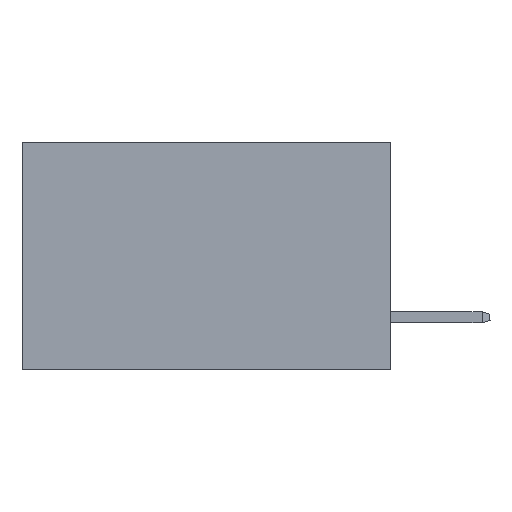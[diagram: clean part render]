
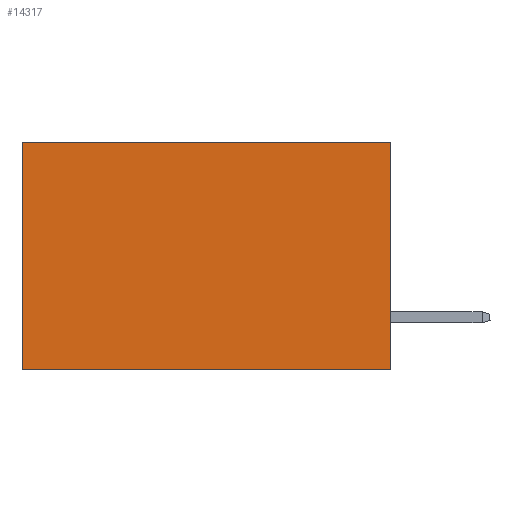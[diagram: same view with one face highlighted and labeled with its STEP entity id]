
A CAD part, left-side view. The second image highlights one B-rep face of the part: STEP entity #14317.
In plain terms, the highlighted planar face has unit normal (-1, 0, 0).
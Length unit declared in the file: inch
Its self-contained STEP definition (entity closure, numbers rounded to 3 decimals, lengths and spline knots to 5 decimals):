
#1165 = EDGE_CURVE ( 'NONE', #21384, #20800, #18190, .T. ) ;
#1478 = CARTESIAN_POINT ( 'NONE',  ( 0.2875, 0., 0. ) ) ;
#1890 = FACE_OUTER_BOUND ( 'NONE', #25519, .T. ) ;
#4915 = ORIENTED_EDGE ( 'NONE', *, *, #15738, .F. ) ;
#5184 = DIRECTION ( 'NONE',  ( 1., 0., 0. ) ) ;
#6334 = CARTESIAN_POINT ( 'NONE',  ( 0.2875, 0.6, 0. ) ) ;
#7703 = LINE ( 'NONE', #1478, #8691 ) ;
#8682 = VERTEX_POINT ( 'NONE', #22305 ) ;
#8691 = VECTOR ( 'NONE', #23626, 39.37008 ) ;
#9020 = ORIENTED_EDGE ( 'NONE', *, *, #1165, .T. ) ;
#9028 = PLANE ( 'NONE',  #11332 ) ;
#10023 = CARTESIAN_POINT ( 'NONE',  ( 0.2875, 0., 0. ) ) ;
#10754 = CARTESIAN_POINT ( 'NONE',  ( 0.2875, 0., 0. ) ) ;
#11332 = AXIS2_PLACEMENT_3D ( 'NONE', #13520, #5184, #19682 ) ;
#11790 = ORIENTED_EDGE ( 'NONE', *, *, #26344, .F. ) ;
#11965 = CARTESIAN_POINT ( 'NONE',  ( 0.2875, 0.6, 0. ) ) ;
#12407 = VECTOR ( 'NONE', #26086, 39.37008 ) ;
#13243 = ORIENTED_EDGE ( 'NONE', *, *, #21626, .T. ) ;
#13520 = CARTESIAN_POINT ( 'NONE',  ( 0.2875, 0., 0. ) ) ;
#14317 = ADVANCED_FACE ( 'NONE', ( #1890 ), #9028, .F. ) ;
#14984 = LINE ( 'NONE', #23029, #24853 ) ;
#15738 = EDGE_CURVE ( 'NONE', #8682, #24709, #14984, .T. ) ;
#15828 = LINE ( 'NONE', #11965, #16168 ) ;
#16168 = VECTOR ( 'NONE', #22227, 39.37008 ) ;
#16322 = CARTESIAN_POINT ( 'NONE',  ( 0.2875, 0.6, -0.37 ) ) ;
#17677 = DIRECTION ( 'NONE',  ( 0., 1., 0. ) ) ;
#18190 = LINE ( 'NONE', #10023, #12407 ) ;
#19682 = DIRECTION ( 'NONE',  ( 0., 0., -1. ) ) ;
#20800 = VERTEX_POINT ( 'NONE', #6334 ) ;
#21384 = VERTEX_POINT ( 'NONE', #10754 ) ;
#21626 = EDGE_CURVE ( 'NONE', #20800, #24709, #15828, .T. ) ;
#22227 = DIRECTION ( 'NONE',  ( 0., 0., -1. ) ) ;
#22305 = CARTESIAN_POINT ( 'NONE',  ( 0.2875, 0., -0.37 ) ) ;
#23029 = CARTESIAN_POINT ( 'NONE',  ( 0.2875, 0., -0.37 ) ) ;
#23626 = DIRECTION ( 'NONE',  ( 0., 0., -1. ) ) ;
#24709 = VERTEX_POINT ( 'NONE', #16322 ) ;
#24853 = VECTOR ( 'NONE', #17677, 39.37008 ) ;
#25519 = EDGE_LOOP ( 'NONE', ( #13243, #4915, #11790, #9020 ) ) ;
#26086 = DIRECTION ( 'NONE',  ( 0., 1., 0. ) ) ;
#26344 = EDGE_CURVE ( 'NONE', #21384, #8682, #7703, .T. ) ;
